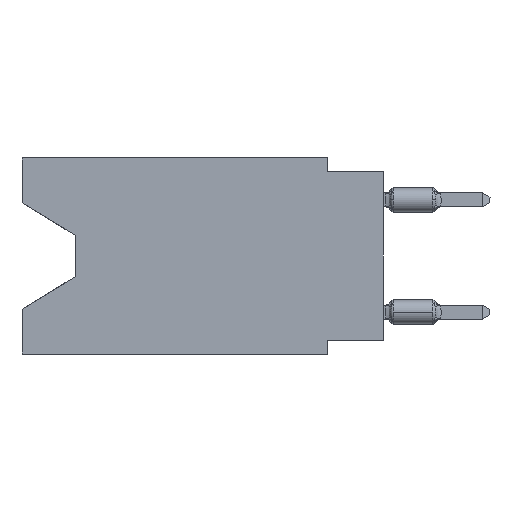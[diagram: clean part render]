
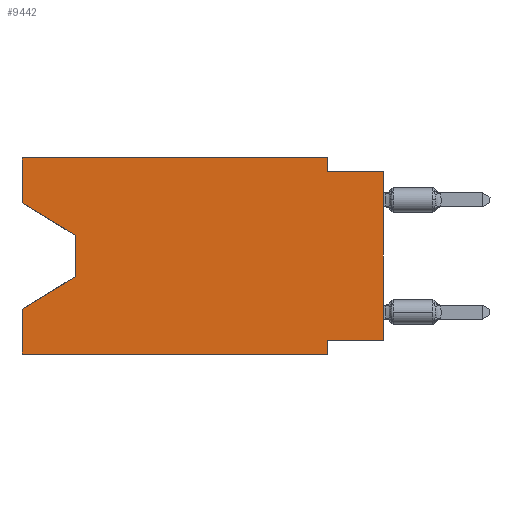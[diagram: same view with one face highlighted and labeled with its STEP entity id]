
A CAD part, left-side view. The second image highlights one B-rep face of the part: STEP entity #9442.
In plain terms, the highlighted planar face has unit normal (-1, 0, 0).
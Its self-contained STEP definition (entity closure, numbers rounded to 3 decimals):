
#28 = EDGE_CURVE ( 'NONE', #10283, #6248, #11749, .T. ) ;
#188 = VECTOR ( 'NONE', #13151, 1000. ) ;
#301 = ORIENTED_EDGE ( 'NONE', *, *, #1030, .F. ) ;
#354 = VECTOR ( 'NONE', #10725, 1000. ) ;
#448 = EDGE_CURVE ( 'NONE', #10283, #1270, #4335, .T. ) ;
#818 = CARTESIAN_POINT ( 'NONE',  ( 0., 0., -0.635 ) ) ;
#1030 = EDGE_CURVE ( 'NONE', #1408, #6248, #4388, .T. ) ;
#1270 = VERTEX_POINT ( 'NONE', #2939 ) ;
#1353 = CARTESIAN_POINT ( 'NONE',  ( 0., 16.383, -2.038 ) ) ;
#1372 = DIRECTION ( 'NONE',  ( 0., 0.855, -0.519 ) ) ;
#1408 = VERTEX_POINT ( 'NONE', #5332 ) ;
#1820 = VECTOR ( 'NONE', #9773, 1000. ) ;
#2443 = VECTOR ( 'NONE', #11505, 1000. ) ;
#2508 = ORIENTED_EDGE ( 'NONE', *, *, #9152, .T. ) ;
#2662 = DIRECTION ( 'NONE',  ( 0., -0.855, -0.519 ) ) ;
#2717 = VECTOR ( 'NONE', #12421, 1000. ) ;
#2765 = EDGE_CURVE ( 'NONE', #6954, #9095, #8899, .T. ) ;
#2939 = CARTESIAN_POINT ( 'NONE',  ( 0., 16.383, -6.852 ) ) ;
#3129 = CARTESIAN_POINT ( 'NONE',  ( 0., 13.97, -3.505 ) ) ;
#3303 = DIRECTION ( 'NONE',  ( 0., 0., -1. ) ) ;
#3335 = LINE ( 'NONE', #8754, #1820 ) ;
#3442 = LINE ( 'NONE', #4665, #11033 ) ;
#3473 = VECTOR ( 'NONE', #3303, 1000. ) ;
#3477 = ORIENTED_EDGE ( 'NONE', *, *, #5140, .F. ) ;
#3592 = AXIS2_PLACEMENT_3D ( 'NONE', #8950, #8813, #3803 ) ;
#3642 = DIRECTION ( 'NONE',  ( 0., 0., 1. ) ) ;
#3803 = DIRECTION ( 'NONE',  ( 0., 0., -1. ) ) ;
#4089 = ORIENTED_EDGE ( 'NONE', *, *, #10440, .F. ) ;
#4206 = ORIENTED_EDGE ( 'NONE', *, *, #28, .T. ) ;
#4330 = LINE ( 'NONE', #12676, #3473 ) ;
#4335 = LINE ( 'NONE', #11592, #7384 ) ;
#4388 = LINE ( 'NONE', #12727, #2443 ) ;
#4418 = CARTESIAN_POINT ( 'NONE',  ( 0., 2.54, -8.89 ) ) ;
#4440 = VECTOR ( 'NONE', #3642, 1000. ) ;
#4665 = CARTESIAN_POINT ( 'NONE',  ( 0., 16.383, 0. ) ) ;
#4912 = CARTESIAN_POINT ( 'NONE',  ( 0., 13.97, -5.385 ) ) ;
#4921 = VECTOR ( 'NONE', #8390, 1000. ) ;
#4994 = VERTEX_POINT ( 'NONE', #12089 ) ;
#5069 = EDGE_LOOP ( 'NONE', ( #6173, #2508, #13190, #9956, #4206, #301, #4089, #7973, #3477, #6021, #5957, #7845 ) ) ;
#5140 = EDGE_CURVE ( 'NONE', #9347, #11519, #11462, .T. ) ;
#5239 = CARTESIAN_POINT ( 'NONE',  ( 0., 0., -0.635 ) ) ;
#5332 = CARTESIAN_POINT ( 'NONE',  ( 0., 2.54, -8.255 ) ) ;
#5591 = EDGE_CURVE ( 'NONE', #6954, #5902, #3442, .T. ) ;
#5720 = CARTESIAN_POINT ( 'NONE',  ( 0., 2.54, -0.635 ) ) ;
#5902 = VERTEX_POINT ( 'NONE', #12510 ) ;
#5917 = CARTESIAN_POINT ( 'NONE',  ( 0., 16.383, 0. ) ) ;
#5957 = ORIENTED_EDGE ( 'NONE', *, *, #13117, .F. ) ;
#6021 = ORIENTED_EDGE ( 'NONE', *, *, #13406, .F. ) ;
#6173 = ORIENTED_EDGE ( 'NONE', *, *, #2765, .T. ) ;
#6248 = VERTEX_POINT ( 'NONE', #4418 ) ;
#6486 = CARTESIAN_POINT ( 'NONE',  ( 0., 16.383, -8.89 ) ) ;
#6723 = LINE ( 'NONE', #12047, #4440 ) ;
#6954 = VERTEX_POINT ( 'NONE', #9184 ) ;
#7384 = VECTOR ( 'NONE', #9546, 1000. ) ;
#7616 = CARTESIAN_POINT ( 'NONE',  ( 0., 13.97, -5.385 ) ) ;
#7845 = ORIENTED_EDGE ( 'NONE', *, *, #5591, .F. ) ;
#7917 = FACE_OUTER_BOUND ( 'NONE', #5069, .T. ) ;
#7973 = ORIENTED_EDGE ( 'NONE', *, *, #11408, .T. ) ;
#8390 = DIRECTION ( 'NONE',  ( 0., -1., 0. ) ) ;
#8552 = VERTEX_POINT ( 'NONE', #9930 ) ;
#8754 = CARTESIAN_POINT ( 'NONE',  ( 0., 0., -8.255 ) ) ;
#8813 = DIRECTION ( 'NONE',  ( 1., 0., 0. ) ) ;
#8851 = LINE ( 'NONE', #7616, #13052 ) ;
#8899 = LINE ( 'NONE', #1353, #10042 ) ;
#8950 = CARTESIAN_POINT ( 'NONE',  ( 0., 16.383, 0. ) ) ;
#8988 = VERTEX_POINT ( 'NONE', #4912 ) ;
#9095 = VERTEX_POINT ( 'NONE', #9294 ) ;
#9152 = EDGE_CURVE ( 'NONE', #9095, #8988, #12356, .T. ) ;
#9184 = CARTESIAN_POINT ( 'NONE',  ( 0., 16.383, -2.038 ) ) ;
#9294 = CARTESIAN_POINT ( 'NONE',  ( 0., 13.97, -3.505 ) ) ;
#9347 = VERTEX_POINT ( 'NONE', #5720 ) ;
#9442 = ADVANCED_FACE ( 'NONE', ( #7917 ), #10865, .F. ) ;
#9546 = DIRECTION ( 'NONE',  ( 0., 0., 1. ) ) ;
#9773 = DIRECTION ( 'NONE',  ( 0., 1., 0. ) ) ;
#9930 = CARTESIAN_POINT ( 'NONE',  ( 0., 0., -8.255 ) ) ;
#9956 = ORIENTED_EDGE ( 'NONE', *, *, #448, .F. ) ;
#10042 = VECTOR ( 'NONE', #2662, 1000. ) ;
#10161 = LINE ( 'NONE', #5917, #188 ) ;
#10283 = VERTEX_POINT ( 'NONE', #11481 ) ;
#10440 = EDGE_CURVE ( 'NONE', #8552, #1408, #3335, .T. ) ;
#10725 = DIRECTION ( 'NONE',  ( 0., -1., 0. ) ) ;
#10865 = PLANE ( 'NONE',  #3592 ) ;
#10904 = DIRECTION ( 'NONE',  ( 0., 0., 1. ) ) ;
#11033 = VECTOR ( 'NONE', #10904, 1000. ) ;
#11408 = EDGE_CURVE ( 'NONE', #8552, #11519, #6723, .T. ) ;
#11462 = LINE ( 'NONE', #5239, #4921 ) ;
#11481 = CARTESIAN_POINT ( 'NONE',  ( 0., 16.383, -8.89 ) ) ;
#11505 = DIRECTION ( 'NONE',  ( 0., 0., -1. ) ) ;
#11519 = VERTEX_POINT ( 'NONE', #818 ) ;
#11592 = CARTESIAN_POINT ( 'NONE',  ( 0., 16.383, 0. ) ) ;
#11749 = LINE ( 'NONE', #6486, #354 ) ;
#12047 = CARTESIAN_POINT ( 'NONE',  ( 0., 0., 0. ) ) ;
#12089 = CARTESIAN_POINT ( 'NONE',  ( 0., 2.54, 0. ) ) ;
#12224 = EDGE_CURVE ( 'NONE', #8988, #1270, #8851, .T. ) ;
#12356 = LINE ( 'NONE', #3129, #2717 ) ;
#12421 = DIRECTION ( 'NONE',  ( 0., 0., -1. ) ) ;
#12510 = CARTESIAN_POINT ( 'NONE',  ( 0., 16.383, 0. ) ) ;
#12676 = CARTESIAN_POINT ( 'NONE',  ( 0., 2.54, 0. ) ) ;
#12727 = CARTESIAN_POINT ( 'NONE',  ( 0., 2.54, -8.89 ) ) ;
#13052 = VECTOR ( 'NONE', #1372, 1000. ) ;
#13117 = EDGE_CURVE ( 'NONE', #5902, #4994, #10161, .T. ) ;
#13151 = DIRECTION ( 'NONE',  ( 0., -1., 0. ) ) ;
#13190 = ORIENTED_EDGE ( 'NONE', *, *, #12224, .T. ) ;
#13406 = EDGE_CURVE ( 'NONE', #4994, #9347, #4330, .T. ) ;
